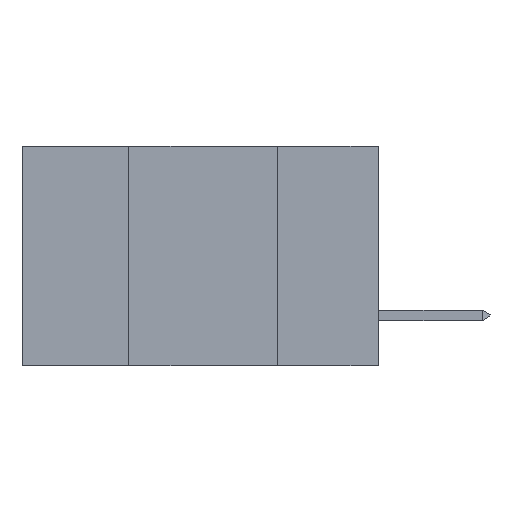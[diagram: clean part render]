
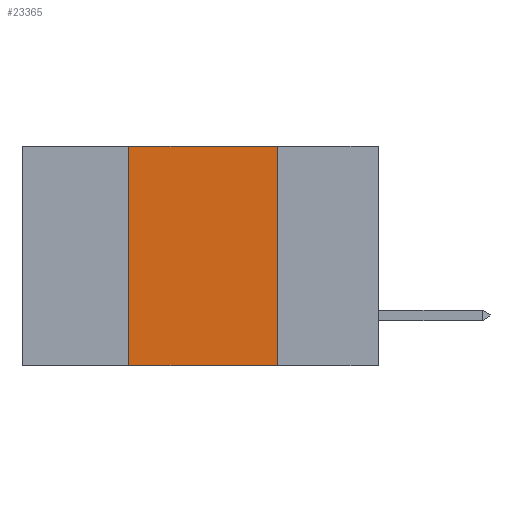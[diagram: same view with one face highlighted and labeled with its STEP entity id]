
A CAD part, left-side view. The second image highlights one B-rep face of the part: STEP entity #23365.
In plain terms, the highlighted planar face has unit normal (-1, 0, 0).
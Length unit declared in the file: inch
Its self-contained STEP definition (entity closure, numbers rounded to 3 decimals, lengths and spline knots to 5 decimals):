
#401 = LINE ( 'NONE', #4675, #12011 ) ;
#663 = DIRECTION ( 'NONE',  ( 0., -1., 0. ) ) ;
#2373 = VERTEX_POINT ( 'NONE', #9835 ) ;
#3393 = CARTESIAN_POINT ( 'NONE',  ( 0., 0.42, -0.37 ) ) ;
#4675 = CARTESIAN_POINT ( 'NONE',  ( 0., 0.6, -0.37 ) ) ;
#4753 = VERTEX_POINT ( 'NONE', #9087 ) ;
#6288 = CARTESIAN_POINT ( 'NONE',  ( 0., 0.6, 0. ) ) ;
#6846 = EDGE_LOOP ( 'NONE', ( #7776, #21726, #7690, #7390 ) ) ;
#7390 = ORIENTED_EDGE ( 'NONE', *, *, #24525, .T. ) ;
#7671 = CARTESIAN_POINT ( 'NONE',  ( 0., 0.42, -0.37 ) ) ;
#7690 = ORIENTED_EDGE ( 'NONE', *, *, #17466, .F. ) ;
#7698 = CARTESIAN_POINT ( 'NONE',  ( 0., 0.6, 0. ) ) ;
#7776 = ORIENTED_EDGE ( 'NONE', *, *, #25262, .F. ) ;
#9087 = CARTESIAN_POINT ( 'NONE',  ( 0., 0.17, -0.37 ) ) ;
#9808 = DIRECTION ( 'NONE',  ( 0., -1., 0. ) ) ;
#9835 = CARTESIAN_POINT ( 'NONE',  ( 0., 0.42, 0. ) ) ;
#10756 = VECTOR ( 'NONE', #22009, 39.37008 ) ;
#10803 = FACE_OUTER_BOUND ( 'NONE', #6846, .T. ) ;
#11575 = LINE ( 'NONE', #21877, #10756 ) ;
#11858 = EDGE_CURVE ( 'NONE', #2373, #22014, #19588, .T. ) ;
#12011 = VECTOR ( 'NONE', #663, 39.37008 ) ;
#13213 = VECTOR ( 'NONE', #19707, 39.37008 ) ;
#13547 = VERTEX_POINT ( 'NONE', #7671 ) ;
#14938 = DIRECTION ( 'NONE',  ( 0., 0., -1. ) ) ;
#15875 = AXIS2_PLACEMENT_3D ( 'NONE', #6288, #16961, #14938 ) ;
#16961 = DIRECTION ( 'NONE',  ( 1., 0., 0. ) ) ;
#17466 = EDGE_CURVE ( 'NONE', #13547, #2373, #19434, .T. ) ;
#19434 = LINE ( 'NONE', #3393, #13213 ) ;
#19588 = LINE ( 'NONE', #7698, #21192 ) ;
#19707 = DIRECTION ( 'NONE',  ( 0., 0., 1. ) ) ;
#21192 = VECTOR ( 'NONE', #9808, 39.37008 ) ;
#21726 = ORIENTED_EDGE ( 'NONE', *, *, #11858, .F. ) ;
#21877 = CARTESIAN_POINT ( 'NONE',  ( 0., 0.17, -0.37 ) ) ;
#22009 = DIRECTION ( 'NONE',  ( 0., 0., -1. ) ) ;
#22014 = VERTEX_POINT ( 'NONE', #26141 ) ;
#23365 = ADVANCED_FACE ( 'NONE', ( #10803 ), #25125, .F. ) ;
#24525 = EDGE_CURVE ( 'NONE', #13547, #4753, #401, .T. ) ;
#25125 = PLANE ( 'NONE',  #15875 ) ;
#25262 = EDGE_CURVE ( 'NONE', #22014, #4753, #11575, .T. ) ;
#26141 = CARTESIAN_POINT ( 'NONE',  ( 0., 0.17, 0. ) ) ;
